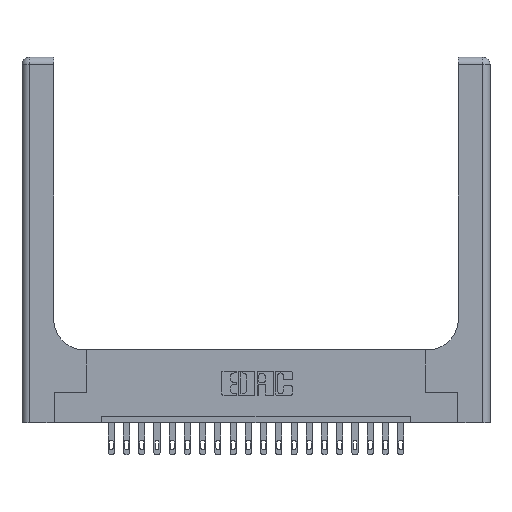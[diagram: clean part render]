
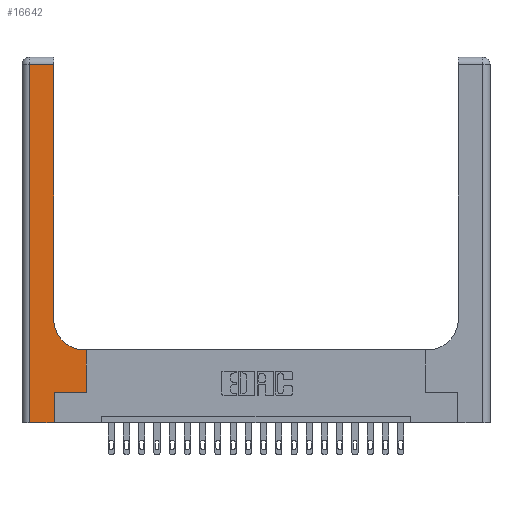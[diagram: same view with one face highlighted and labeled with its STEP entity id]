
A CAD part, top view. The second image highlights one B-rep face of the part: STEP entity #16642.
In plain terms, the highlighted planar face has unit normal (0, 0, 1).
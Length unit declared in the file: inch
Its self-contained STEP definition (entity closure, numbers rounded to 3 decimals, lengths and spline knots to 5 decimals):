
#20 = CARTESIAN_POINT ( 'NONE',  ( 0.265, 0.25, 0.37 ) ) ;
#216 = CARTESIAN_POINT ( 'NONE',  ( 0.528, 0.25, 0.37 ) ) ;
#519 = LINE ( 'NONE', #3826, #5974 ) ;
#740 = DIRECTION ( 'NONE',  ( 0., 1., 0. ) ) ;
#879 = LINE ( 'NONE', #12224, #18559 ) ;
#1932 = DIRECTION ( 'NONE',  ( 0., 0., -1. ) ) ;
#2681 = ORIENTED_EDGE ( 'NONE', *, *, #17675, .T. ) ;
#2724 = VECTOR ( 'NONE', #5386, 39.37008 ) ;
#3103 = DIRECTION ( 'NONE',  ( -1., 0., 0. ) ) ;
#3375 = LINE ( 'NONE', #19741, #2724 ) ;
#3746 = AXIS2_PLACEMENT_3D ( 'NONE', #13249, #1932, #15271 ) ;
#3778 = ORIENTED_EDGE ( 'NONE', *, *, #9392, .T. ) ;
#3826 = CARTESIAN_POINT ( 'NONE',  ( 0.265, 0., 0.37 ) ) ;
#3871 = ORIENTED_EDGE ( 'NONE', *, *, #13296, .T. ) ;
#4252 = DIRECTION ( 'NONE',  ( 0., -1., 0. ) ) ;
#4328 = DIRECTION ( 'NONE',  ( -1., 0., 0. ) ) ;
#4655 = ORIENTED_EDGE ( 'NONE', *, *, #9264, .T. ) ;
#5323 = LINE ( 'NONE', #11659, #13145 ) ;
#5335 = CARTESIAN_POINT ( 'NONE',  ( 0.06, 3., 0.37 ) ) ;
#5386 = DIRECTION ( 'NONE',  ( -1., 0., 0. ) ) ;
#5651 = EDGE_CURVE ( 'NONE', #6067, #19810, #20213, .T. ) ;
#5745 = ORIENTED_EDGE ( 'NONE', *, *, #10027, .T. ) ;
#5910 = PLANE ( 'NONE',  #13646 ) ;
#5943 = CARTESIAN_POINT ( 'NONE',  ( 0.26, 3., 0.37 ) ) ;
#5974 = VECTOR ( 'NONE', #20101, 39.37008 ) ;
#6067 = VERTEX_POINT ( 'NONE', #7582 ) ;
#6311 = ORIENTED_EDGE ( 'NONE', *, *, #7668, .T. ) ;
#7433 = EDGE_LOOP ( 'NONE', ( #11267, #19209, #6311, #3778, #2681, #4655, #5745, #12274, #3871 ) ) ;
#7582 = CARTESIAN_POINT ( 'NONE',  ( 0.26, 0.85, 0.37 ) ) ;
#7668 = EDGE_CURVE ( 'NONE', #19183, #12227, #18720, .T. ) ;
#7681 = VERTEX_POINT ( 'NONE', #9980 ) ;
#8074 = EDGE_CURVE ( 'NONE', #19810, #19183, #15906, .T. ) ;
#9264 = EDGE_CURVE ( 'NONE', #9508, #11911, #879, .T. ) ;
#9356 = VERTEX_POINT ( 'NONE', #20770 ) ;
#9392 = EDGE_CURVE ( 'NONE', #12227, #9356, #5323, .T. ) ;
#9508 = VERTEX_POINT ( 'NONE', #20 ) ;
#9511 = CIRCLE ( 'NONE', #3746, 0.25 ) ;
#9980 = CARTESIAN_POINT ( 'NONE',  ( 0.528, 0.6, 0.37 ) ) ;
#10004 = VECTOR ( 'NONE', #740, 39.37008 ) ;
#10027 = EDGE_CURVE ( 'NONE', #11911, #7681, #16584, .T. ) ;
#10489 = VECTOR ( 'NONE', #16798, 39.37008 ) ;
#11267 = ORIENTED_EDGE ( 'NONE', *, *, #5651, .T. ) ;
#11361 = CARTESIAN_POINT ( 'NONE',  ( 0.51, 0.6, 0.37 ) ) ;
#11421 = CARTESIAN_POINT ( 'NONE',  ( 0.06, 2.94, 0.37 ) ) ;
#11659 = CARTESIAN_POINT ( 'NONE',  ( 0., 0., 0.37 ) ) ;
#11911 = VERTEX_POINT ( 'NONE', #216 ) ;
#12065 = CARTESIAN_POINT ( 'NONE',  ( 0.528, 0.25, 0.37 ) ) ;
#12224 = CARTESIAN_POINT ( 'NONE',  ( 0.265, 0.25, 0.37 ) ) ;
#12227 = VERTEX_POINT ( 'NONE', #15786 ) ;
#12274 = ORIENTED_EDGE ( 'NONE', *, *, #12824, .T. ) ;
#12352 = CARTESIAN_POINT ( 'NONE',  ( 0., 3., 0.37 ) ) ;
#12824 = EDGE_CURVE ( 'NONE', #7681, #15901, #3375, .T. ) ;
#13145 = VECTOR ( 'NONE', #16102, 39.37008 ) ;
#13249 = CARTESIAN_POINT ( 'NONE',  ( 0.51, 0.85, 0.37 ) ) ;
#13296 = EDGE_CURVE ( 'NONE', #15901, #6067, #9511, .T. ) ;
#13646 = AXIS2_PLACEMENT_3D ( 'NONE', #12352, #18791, #4328 ) ;
#14122 = VECTOR ( 'NONE', #4252, 39.37008 ) ;
#14306 = CARTESIAN_POINT ( 'NONE',  ( 0., 2.94, 0.37 ) ) ;
#14590 = CARTESIAN_POINT ( 'NONE',  ( 0.26, 2.94, 0.37 ) ) ;
#15271 = DIRECTION ( 'NONE',  ( 1., 0., 0. ) ) ;
#15786 = CARTESIAN_POINT ( 'NONE',  ( 0.06, 0., 0.37 ) ) ;
#15901 = VERTEX_POINT ( 'NONE', #11361 ) ;
#15906 = LINE ( 'NONE', #14306, #19854 ) ;
#16102 = DIRECTION ( 'NONE',  ( 1., 0., 0. ) ) ;
#16584 = LINE ( 'NONE', #12065, #10489 ) ;
#16642 = ADVANCED_FACE ( 'NONE', ( #17403 ), #5910, .F. ) ;
#16798 = DIRECTION ( 'NONE',  ( 0., 1., 0. ) ) ;
#17403 = FACE_OUTER_BOUND ( 'NONE', #7433, .T. ) ;
#17675 = EDGE_CURVE ( 'NONE', #9356, #9508, #519, .T. ) ;
#18559 = VECTOR ( 'NONE', #20141, 39.37008 ) ;
#18720 = LINE ( 'NONE', #5335, #14122 ) ;
#18791 = DIRECTION ( 'NONE',  ( 0., 0., -1. ) ) ;
#19183 = VERTEX_POINT ( 'NONE', #11421 ) ;
#19209 = ORIENTED_EDGE ( 'NONE', *, *, #8074, .T. ) ;
#19741 = CARTESIAN_POINT ( 'NONE',  ( 0.26, 0.6, 0.37 ) ) ;
#19810 = VERTEX_POINT ( 'NONE', #14590 ) ;
#19854 = VECTOR ( 'NONE', #3103, 39.37008 ) ;
#20101 = DIRECTION ( 'NONE',  ( 0., 1., 0. ) ) ;
#20141 = DIRECTION ( 'NONE',  ( 1., 0., 0. ) ) ;
#20213 = LINE ( 'NONE', #5943, #10004 ) ;
#20770 = CARTESIAN_POINT ( 'NONE',  ( 0.265, 0., 0.37 ) ) ;
